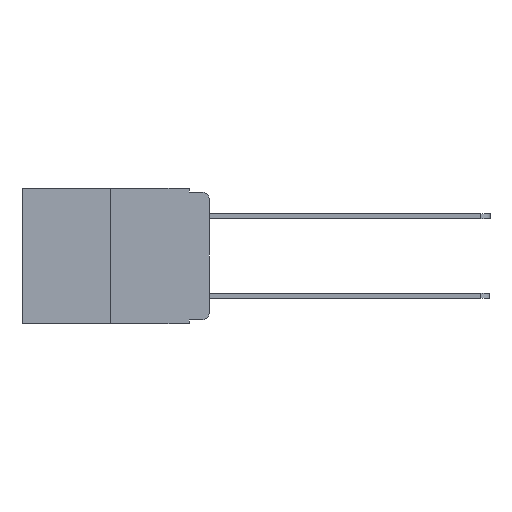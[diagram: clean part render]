
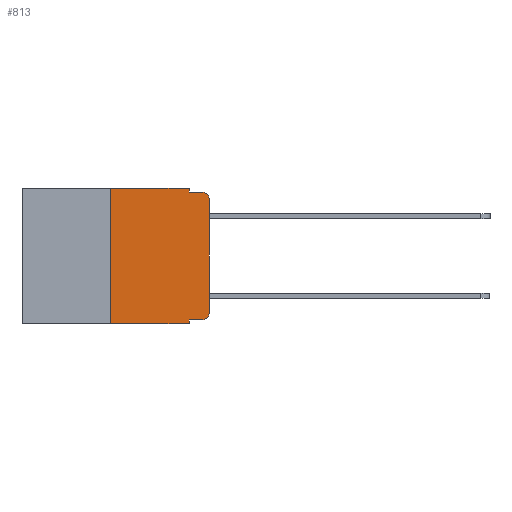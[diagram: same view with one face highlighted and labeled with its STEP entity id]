
A CAD part, left-side view. The second image highlights one B-rep face of the part: STEP entity #813.
In plain terms, the highlighted planar face has unit normal (-1, 0, 0).
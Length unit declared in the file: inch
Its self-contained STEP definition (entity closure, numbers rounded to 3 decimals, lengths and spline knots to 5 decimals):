
#219 = CARTESIAN_POINT ( 'NONE',  ( 0., 0.02, -0.333 ) ) ;
#411 = AXIS2_PLACEMENT_3D ( 'NONE', #7150, #8423, #5953 ) ;
#754 = ORIENTED_EDGE ( 'NONE', *, *, #6975, .F. ) ;
#792 = EDGE_CURVE ( 'NONE', #4660, #8160, #2958, .T. ) ;
#813 = ADVANCED_FACE ( 'NONE', ( #2703 ), #1780, .F. ) ;
#924 = EDGE_CURVE ( 'NONE', #9606, #2870, #3883, .T. ) ;
#1018 = VECTOR ( 'NONE', #1055, 39.37008 ) ;
#1055 = DIRECTION ( 'NONE',  ( 0., 0., 1. ) ) ;
#1211 = LINE ( 'NONE', #3518, #7680 ) ;
#1357 = ORIENTED_EDGE ( 'NONE', *, *, #7994, .T. ) ;
#1564 = AXIS2_PLACEMENT_3D ( 'NONE', #9525, #8738, #5380 ) ;
#1641 = DIRECTION ( 'NONE',  ( 0., -1., 0. ) ) ;
#1701 = ORIENTED_EDGE ( 'NONE', *, *, #9048, .F. ) ;
#1780 = PLANE ( 'NONE',  #9750 ) ;
#1851 = CIRCLE ( 'NONE', #411, 0.02 ) ;
#1938 = VERTEX_POINT ( 'NONE', #4983 ) ;
#1988 = LINE ( 'NONE', #8514, #8725 ) ;
#2113 = ORIENTED_EDGE ( 'NONE', *, *, #2707, .T. ) ;
#2171 = DIRECTION ( 'NONE',  ( 0., -1., 0. ) ) ;
#2276 = EDGE_CURVE ( 'NONE', #4043, #1938, #1988, .T. ) ;
#2314 = CARTESIAN_POINT ( 'NONE',  ( 0., 0.051, -0.01 ) ) ;
#2571 = EDGE_CURVE ( 'NONE', #8160, #6470, #1851, .T. ) ;
#2703 = FACE_OUTER_BOUND ( 'NONE', #6847, .T. ) ;
#2707 = EDGE_CURVE ( 'NONE', #5530, #10099, #2787, .T. ) ;
#2787 = CIRCLE ( 'NONE', #1564, 0.02 ) ;
#2870 = VERTEX_POINT ( 'NONE', #7060 ) ;
#2958 = LINE ( 'NONE', #8546, #7186 ) ;
#3106 = CARTESIAN_POINT ( 'NONE',  ( 0., 0.051, 0. ) ) ;
#3391 = CARTESIAN_POINT ( 'NONE',  ( 0., 0., 0. ) ) ;
#3518 = CARTESIAN_POINT ( 'NONE',  ( 0., 0.051, 0. ) ) ;
#3627 = VECTOR ( 'NONE', #10018, 39.37008 ) ;
#3883 = LINE ( 'NONE', #8146, #10248 ) ;
#4043 = VERTEX_POINT ( 'NONE', #6667 ) ;
#4092 = ORIENTED_EDGE ( 'NONE', *, *, #9524, .F. ) ;
#4660 = VERTEX_POINT ( 'NONE', #6531 ) ;
#4846 = CARTESIAN_POINT ( 'NONE',  ( 0., 0., -0.03 ) ) ;
#4860 = CARTESIAN_POINT ( 'NONE',  ( 0., 0., -0.313 ) ) ;
#4983 = CARTESIAN_POINT ( 'NONE',  ( 0., 0.051, 0. ) ) ;
#5286 = CARTESIAN_POINT ( 'NONE',  ( 0., 0.25, 0. ) ) ;
#5380 = DIRECTION ( 'NONE',  ( 0., 0., -1. ) ) ;
#5530 = VERTEX_POINT ( 'NONE', #4846 ) ;
#5737 = DIRECTION ( 'NONE',  ( 0., -1., 0. ) ) ;
#5953 = DIRECTION ( 'NONE',  ( 0., 0., -1. ) ) ;
#6106 = DIRECTION ( 'NONE',  ( 0., 0., -1. ) ) ;
#6279 = VECTOR ( 'NONE', #8995, 39.37008 ) ;
#6337 = ORIENTED_EDGE ( 'NONE', *, *, #2276, .F. ) ;
#6470 = VERTEX_POINT ( 'NONE', #4860 ) ;
#6531 = CARTESIAN_POINT ( 'NONE',  ( 0., 0.051, -0.333 ) ) ;
#6586 = VECTOR ( 'NONE', #2171, 39.37008 ) ;
#6667 = CARTESIAN_POINT ( 'NONE',  ( 0., 0.25, 0. ) ) ;
#6697 = ORIENTED_EDGE ( 'NONE', *, *, #2571, .T. ) ;
#6726 = ORIENTED_EDGE ( 'NONE', *, *, #924, .T. ) ;
#6847 = EDGE_LOOP ( 'NONE', ( #1357, #2113, #8273, #4092, #6337, #754, #6726, #1701, #6862, #6697 ) ) ;
#6862 = ORIENTED_EDGE ( 'NONE', *, *, #792, .T. ) ;
#6975 = EDGE_CURVE ( 'NONE', #9606, #4043, #9901, .T. ) ;
#7032 = CARTESIAN_POINT ( 'NONE',  ( 0., 0.25, -0.343 ) ) ;
#7060 = CARTESIAN_POINT ( 'NONE',  ( 0., 0.051, -0.343 ) ) ;
#7091 = DIRECTION ( 'NONE',  ( 0., 0., -1. ) ) ;
#7150 = CARTESIAN_POINT ( 'NONE',  ( 0., 0.02, -0.313 ) ) ;
#7186 = VECTOR ( 'NONE', #1641, 39.37008 ) ;
#7226 = CARTESIAN_POINT ( 'NONE',  ( 0., 0.051, -0.01 ) ) ;
#7680 = VECTOR ( 'NONE', #6106, 39.37008 ) ;
#7923 = CARTESIAN_POINT ( 'NONE',  ( 0., 0.473, 0. ) ) ;
#7994 = EDGE_CURVE ( 'NONE', #6470, #5530, #8099, .T. ) ;
#8099 = LINE ( 'NONE', #3391, #3627 ) ;
#8146 = CARTESIAN_POINT ( 'NONE',  ( 0., 0.473, -0.343 ) ) ;
#8160 = VERTEX_POINT ( 'NONE', #219 ) ;
#8273 = ORIENTED_EDGE ( 'NONE', *, *, #10839, .F. ) ;
#8423 = DIRECTION ( 'NONE',  ( -1., 0., 0. ) ) ;
#8442 = VERTEX_POINT ( 'NONE', #2314 ) ;
#8484 = CARTESIAN_POINT ( 'NONE',  ( 0., 0.02, -0.01 ) ) ;
#8514 = CARTESIAN_POINT ( 'NONE',  ( 0., 0.473, 0. ) ) ;
#8536 = DIRECTION ( 'NONE',  ( 1., 0., 0. ) ) ;
#8546 = CARTESIAN_POINT ( 'NONE',  ( 0., 0.051, -0.333 ) ) ;
#8630 = DIRECTION ( 'NONE',  ( 0., -1., 0. ) ) ;
#8725 = VECTOR ( 'NONE', #8630, 39.37008 ) ;
#8738 = DIRECTION ( 'NONE',  ( -1., 0., 0. ) ) ;
#8806 = LINE ( 'NONE', #7226, #6586 ) ;
#8995 = DIRECTION ( 'NONE',  ( 0., 0., -1. ) ) ;
#9048 = EDGE_CURVE ( 'NONE', #4660, #2870, #10608, .T. ) ;
#9524 = EDGE_CURVE ( 'NONE', #1938, #8442, #1211, .T. ) ;
#9525 = CARTESIAN_POINT ( 'NONE',  ( 0., 0.02, -0.03 ) ) ;
#9606 = VERTEX_POINT ( 'NONE', #7032 ) ;
#9750 = AXIS2_PLACEMENT_3D ( 'NONE', #7923, #8536, #7091 ) ;
#9901 = LINE ( 'NONE', #5286, #1018 ) ;
#10018 = DIRECTION ( 'NONE',  ( 0., 0., 1. ) ) ;
#10099 = VERTEX_POINT ( 'NONE', #8484 ) ;
#10248 = VECTOR ( 'NONE', #5737, 39.37008 ) ;
#10608 = LINE ( 'NONE', #3106, #6279 ) ;
#10839 = EDGE_CURVE ( 'NONE', #8442, #10099, #8806, .T. ) ;
